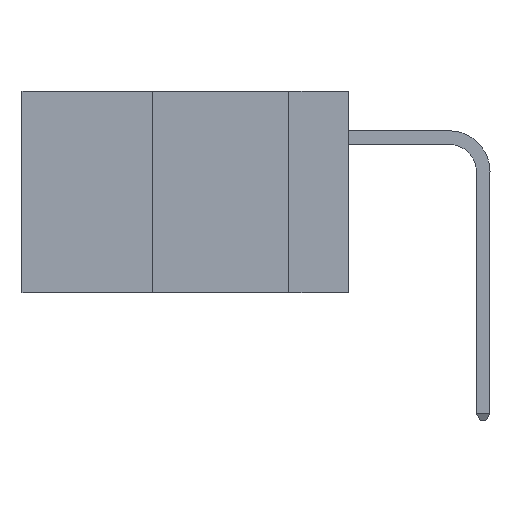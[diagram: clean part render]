
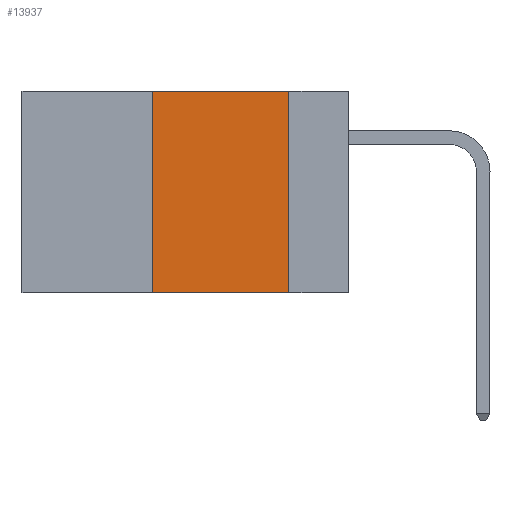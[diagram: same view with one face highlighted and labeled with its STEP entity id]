
A CAD part, left-side view. The second image highlights one B-rep face of the part: STEP entity #13937.
In plain terms, the highlighted planar face has unit normal (-1, 0, 0).
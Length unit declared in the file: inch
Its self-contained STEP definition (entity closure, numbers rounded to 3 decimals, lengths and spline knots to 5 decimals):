
#2044 = LINE ( 'NONE', #17254, #10013 ) ;
#2572 = CARTESIAN_POINT ( 'NONE',  ( 0., 0.11, -0.37 ) ) ;
#2653 = ORIENTED_EDGE ( 'NONE', *, *, #13017, .F. ) ;
#2740 = LINE ( 'NONE', #7660, #10703 ) ;
#3736 = VECTOR ( 'NONE', #10070, 39.37008 ) ;
#4474 = CARTESIAN_POINT ( 'NONE',  ( 0., 0.11, 0. ) ) ;
#5057 = LINE ( 'NONE', #7853, #16409 ) ;
#5217 = VERTEX_POINT ( 'NONE', #10149 ) ;
#6346 = DIRECTION ( 'NONE',  ( 0., -1., 0. ) ) ;
#6452 = FACE_OUTER_BOUND ( 'NONE', #15759, .T. ) ;
#7660 = CARTESIAN_POINT ( 'NONE',  ( 0., 0.6, -0.37 ) ) ;
#7853 = CARTESIAN_POINT ( 'NONE',  ( 0., 0.6, 0. ) ) ;
#7959 = LINE ( 'NONE', #14618, #3736 ) ;
#8702 = CARTESIAN_POINT ( 'NONE',  ( 0., 0.36, -0.37 ) ) ;
#10013 = VECTOR ( 'NONE', #15761, 39.37008 ) ;
#10070 = DIRECTION ( 'NONE',  ( 0., 0., -1. ) ) ;
#10149 = CARTESIAN_POINT ( 'NONE',  ( 0., 0.36, 0. ) ) ;
#10703 = VECTOR ( 'NONE', #18336, 39.37008 ) ;
#10928 = DIRECTION ( 'NONE',  ( 0., 0., -1. ) ) ;
#11319 = EDGE_CURVE ( 'NONE', #5217, #13890, #5057, .T. ) ;
#11400 = ORIENTED_EDGE ( 'NONE', *, *, #16841, .F. ) ;
#11451 = ORIENTED_EDGE ( 'NONE', *, *, #12711, .T. ) ;
#12512 = VERTEX_POINT ( 'NONE', #8702 ) ;
#12711 = EDGE_CURVE ( 'NONE', #12512, #14393, #2740, .T. ) ;
#13017 = EDGE_CURVE ( 'NONE', #13890, #14393, #7959, .T. ) ;
#13212 = ORIENTED_EDGE ( 'NONE', *, *, #11319, .F. ) ;
#13890 = VERTEX_POINT ( 'NONE', #4474 ) ;
#13937 = ADVANCED_FACE ( 'NONE', ( #6452 ), #18416, .F. ) ;
#14393 = VERTEX_POINT ( 'NONE', #2572 ) ;
#14618 = CARTESIAN_POINT ( 'NONE',  ( 0., 0.11, 0. ) ) ;
#15409 = CARTESIAN_POINT ( 'NONE',  ( 0., 0.6, 0. ) ) ;
#15759 = EDGE_LOOP ( 'NONE', ( #2653, #13212, #11400, #11451 ) ) ;
#15761 = DIRECTION ( 'NONE',  ( 0., 0., 1. ) ) ;
#16409 = VECTOR ( 'NONE', #6346, 39.37008 ) ;
#16841 = EDGE_CURVE ( 'NONE', #12512, #5217, #2044, .T. ) ;
#17216 = AXIS2_PLACEMENT_3D ( 'NONE', #15409, #19923, #10928 ) ;
#17254 = CARTESIAN_POINT ( 'NONE',  ( 0., 0.36, 0. ) ) ;
#18336 = DIRECTION ( 'NONE',  ( 0., -1., 0. ) ) ;
#18416 = PLANE ( 'NONE',  #17216 ) ;
#19923 = DIRECTION ( 'NONE',  ( 1., 0., 0. ) ) ;
